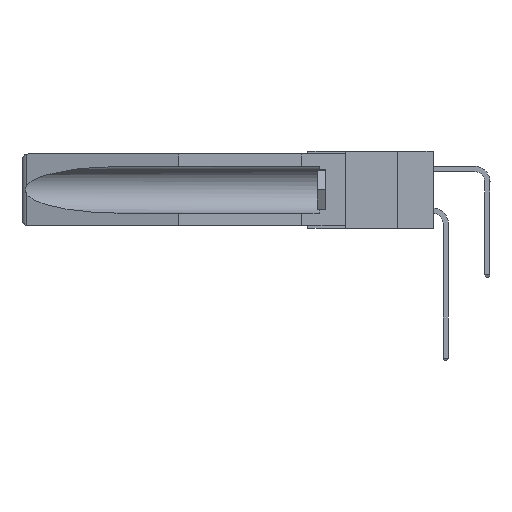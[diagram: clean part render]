
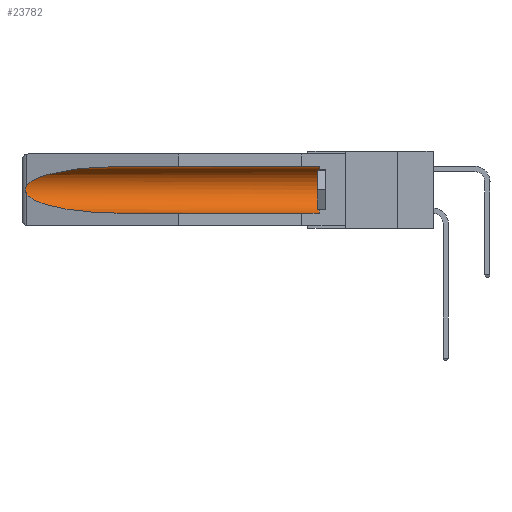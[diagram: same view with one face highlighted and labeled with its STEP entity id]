
A CAD part, left-side view. The second image highlights one B-rep face of the part: STEP entity #23782.
In plain terms, the highlighted cylindrical face has radius 2.857 mm (diameter 5.715 mm), a partial arc.
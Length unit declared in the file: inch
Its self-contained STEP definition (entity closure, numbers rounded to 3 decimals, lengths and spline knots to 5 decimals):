
#339 = EDGE_CURVE ( 'NONE', #11371, #25404, #5290, .T. ) ;
#400 = EDGE_CURVE ( 'NONE', #17108, #2391, #11929, .T. ) ;
#559 = CARTESIAN_POINT ( 'NONE',  ( 0.26537, 1.52718, -0.19328 ) ) ;
#1830 = CARTESIAN_POINT ( 'NONE',  ( 0.155, 1.07973, -0.059 ) ) ;
#1919 = DIRECTION ( 'NONE',  ( 0., 1., 0. ) ) ;
#1948 = CARTESIAN_POINT ( 'NONE',  ( 0.21114, 1.30732, -0.059 ) ) ;
#2391 = VERTEX_POINT ( 'NONE', #29911 ) ;
#2568 = CARTESIAN_POINT ( 'NONE',  ( 0.155, -0.30754, -0.059 ) ) ;
#2839 = CARTESIAN_POINT ( 'NONE',  ( 0.2673, 1.53269, -0.17917 ) ) ;
#3553 =( BOUNDED_CURVE ( )  B_SPLINE_CURVE ( 3, ( #17768, #34208, #31564, #3950 ),
 .UNSPECIFIED., .F., .F. ) 
 B_SPLINE_CURVE_WITH_KNOTS ( ( 4, 4 ),
 ( 0.1948, 1.5708 ),
 .UNSPECIFIED. ) 
 CURVE ( )  GEOMETRIC_REPRESENTATION_ITEM ( )  RATIONAL_B_SPLINE_CURVE ( ( 1., 0.848, 0.848, 1. ) ) 
 REPRESENTATION_ITEM ( '' )  );
#3950 = CARTESIAN_POINT ( 'NONE',  ( 0.155, 1.07973, -0.284 ) ) ;
#4978 = CARTESIAN_POINT ( 'NONE',  ( 0.155, 1.07973, -0.284 ) ) ;
#5091 = FACE_OUTER_BOUND ( 'NONE', #7539, .T. ) ;
#5290 = B_SPLINE_CURVE_WITH_KNOTS ( 'NONE', 3,
 ( #19307, #11400, #30677, #24899, #14145, #25019, #2839, #22076, #33452, #559 ),
 .UNSPECIFIED., .F., .F.,
 ( 4, 2, 2, 2, 4 ),
 ( 0., 0.00029, 0.00058, 0.00087, 0.00117 ),
 .UNSPECIFIED. ) ;
#6849 = VECTOR ( 'NONE', #30619, 39.37008 ) ;
#7036 = EDGE_CURVE ( 'NONE', #25404, #8397, #3553, .T. ) ;
#7539 = EDGE_LOOP ( 'NONE', ( #22852, #24294, #22751, #24229, #19264, #29834 ) ) ;
#7697 = EDGE_CURVE ( 'NONE', #35312, #11371, #34038, .T. ) ;
#8397 = VERTEX_POINT ( 'NONE', #4978 ) ;
#10142 = CARTESIAN_POINT ( 'NONE',  ( 0.25451, 1.48313, -0.09465 ) ) ;
#10558 = CARTESIAN_POINT ( 'NONE',  ( 0.26537, 1.52718, -0.14972 ) ) ;
#11047 = AXIS2_PLACEMENT_3D ( 'NONE', #27681, #25471, #17577 ) ;
#11371 = VERTEX_POINT ( 'NONE', #10558 ) ;
#11400 = CARTESIAN_POINT ( 'NONE',  ( 0.26597, 1.52961, -0.15275 ) ) ;
#11929 = CIRCLE ( 'NONE', #11047, 0.1125 ) ;
#14145 = CARTESIAN_POINT ( 'NONE',  ( 0.2675, 1.53308, -0.16763 ) ) ;
#14238 = LINE ( 'NONE', #27740, #6849 ) ;
#15355 = CARTESIAN_POINT ( 'NONE',  ( 0.155, 1.07973, -0.059 ) ) ;
#17108 = VERTEX_POINT ( 'NONE', #30237 ) ;
#17454 = DIRECTION ( 'NONE',  ( 0., 1., 0. ) ) ;
#17577 = DIRECTION ( 'NONE',  ( 0., 0., 1. ) ) ;
#17768 = CARTESIAN_POINT ( 'NONE',  ( 0.26537, 1.52718, -0.19328 ) ) ;
#19264 = ORIENTED_EDGE ( 'NONE', *, *, #400, .T. ) ;
#19307 = CARTESIAN_POINT ( 'NONE',  ( 0.26537, 1.52718, -0.14972 ) ) ;
#20923 = CARTESIAN_POINT ( 'NONE',  ( 0.155, -0.30754, -0.1715 ) ) ;
#21538 = LINE ( 'NONE', #2568, #33243 ) ;
#22076 = CARTESIAN_POINT ( 'NONE',  ( 0.26655, 1.53094, -0.18657 ) ) ;
#22294 = AXIS2_PLACEMENT_3D ( 'NONE', #20923, #1919, #32073 ) ;
#22751 = ORIENTED_EDGE ( 'NONE', *, *, #7036, .T. ) ;
#22852 = ORIENTED_EDGE ( 'NONE', *, *, #7697, .T. ) ;
#23782 = ADVANCED_FACE ( 'NONE', ( #5091 ), #33589, .F. ) ;
#24229 = ORIENTED_EDGE ( 'NONE', *, *, #28398, .F. ) ;
#24294 = ORIENTED_EDGE ( 'NONE', *, *, #339, .T. ) ;
#24487 = CARTESIAN_POINT ( 'NONE',  ( 0.26537, 1.52718, -0.19328 ) ) ;
#24899 = CARTESIAN_POINT ( 'NONE',  ( 0.2673, 1.5327, -0.16383 ) ) ;
#25019 = CARTESIAN_POINT ( 'NONE',  ( 0.2675, 1.53308, -0.17534 ) ) ;
#25404 = VERTEX_POINT ( 'NONE', #24487 ) ;
#25471 = DIRECTION ( 'NONE',  ( 0., -1., 0. ) ) ;
#27681 = CARTESIAN_POINT ( 'NONE',  ( 0.155, 0.126, -0.1715 ) ) ;
#27740 = CARTESIAN_POINT ( 'NONE',  ( 0.155, -0.30754, -0.284 ) ) ;
#28398 = EDGE_CURVE ( 'NONE', #17108, #8397, #14238, .T. ) ;
#29834 = ORIENTED_EDGE ( 'NONE', *, *, #31064, .T. ) ;
#29911 = CARTESIAN_POINT ( 'NONE',  ( 0.155, 0.126, -0.059 ) ) ;
#30237 = CARTESIAN_POINT ( 'NONE',  ( 0.155, 0.126, -0.284 ) ) ;
#30619 = DIRECTION ( 'NONE',  ( 0., 1., 0. ) ) ;
#30677 = CARTESIAN_POINT ( 'NONE',  ( 0.26654, 1.53092, -0.15636 ) ) ;
#31064 = EDGE_CURVE ( 'NONE', #2391, #35312, #21538, .T. ) ;
#31564 = CARTESIAN_POINT ( 'NONE',  ( 0.21114, 1.30732, -0.284 ) ) ;
#32073 = DIRECTION ( 'NONE',  ( 0., 0., 1. ) ) ;
#32452 = CARTESIAN_POINT ( 'NONE',  ( 0.26537, 1.52718, -0.14972 ) ) ;
#33243 = VECTOR ( 'NONE', #17454, 39.37008 ) ;
#33452 = CARTESIAN_POINT ( 'NONE',  ( 0.26597, 1.5296, -0.19026 ) ) ;
#33589 = CYLINDRICAL_SURFACE ( 'NONE', #22294, 0.1125 ) ;
#34038 =( BOUNDED_CURVE ( )  B_SPLINE_CURVE ( 3, ( #1830, #1948, #10142, #32452 ),
 .UNSPECIFIED., .F., .F. ) 
 B_SPLINE_CURVE_WITH_KNOTS ( ( 4, 4 ),
 ( 4.71239, 6.08839 ),
 .UNSPECIFIED. ) 
 CURVE ( )  GEOMETRIC_REPRESENTATION_ITEM ( )  RATIONAL_B_SPLINE_CURVE ( ( 1., 0.848, 0.848, 1. ) ) 
 REPRESENTATION_ITEM ( '' )  );
#34208 = CARTESIAN_POINT ( 'NONE',  ( 0.25451, 1.48313, -0.24835 ) ) ;
#35312 = VERTEX_POINT ( 'NONE', #15355 ) ;
